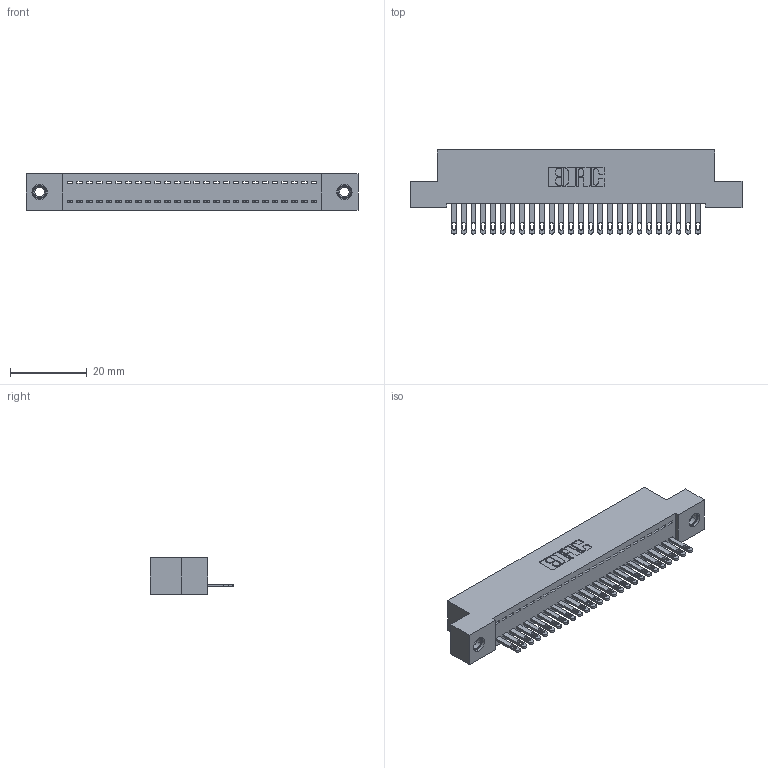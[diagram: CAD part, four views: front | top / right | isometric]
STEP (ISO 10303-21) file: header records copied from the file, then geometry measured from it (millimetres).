
FILE_DESCRIPTION (( 'STEP AP203' ), '1' );
FILE_NAME ('892-026-500-107.STEP', '2020-09-21T14:36:58', ( '' ), ( '' ), 'SwSTEP 2.0', 'SolidWorks 2020', '' );
FILE_SCHEMA (( 'CONFIG_CONTROL_DESIGN' ));
Length unit declared in the file: inch
Products named in the file (4): 842 Part_TI; 345-250-001_345-250-005-103; 345-292-001_345-293-100; 892-026-500-107
Assembly tree (29 placements, depth 2):
  892-026-500-107
    842 Part_TI
    345-292-001_345-293-100  x26
    345-250-001_345-250-005-103  x2
Bounding box: 86.36 x 21.85 x 9.4 mm (x, y, z)
Volume: 7516.5 mm3; surface area: 10822.3 mm2
Topology: 29 solids, 29 shells, 1574 faces, 4803 edges, 3194 vertices
Faces by surface type: plane 1034, cylinder 524, cone 12, torus 4
Entity records: 18948 total; most frequent: CARTESIAN_POINT 3251, ORIENTED_EDGE 3206, DIRECTION 2809, EDGE_CURVE 1603, LINE 1451, VECTOR 1451, VERTEX_POINT 1064, AXIS2_PLACEMENT_3D 679
